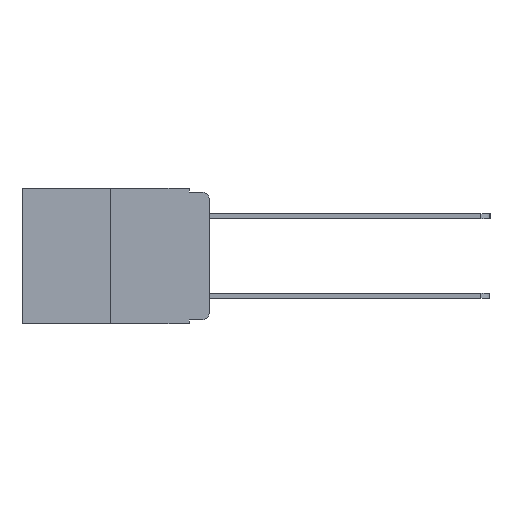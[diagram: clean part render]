
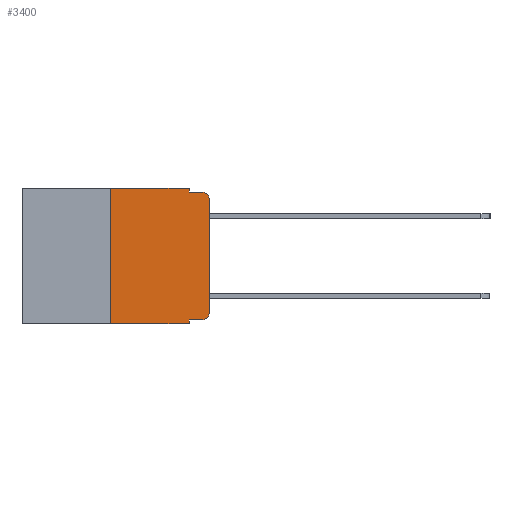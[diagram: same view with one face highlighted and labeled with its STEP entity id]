
A CAD part, left-side view. The second image highlights one B-rep face of the part: STEP entity #3400.
In plain terms, the highlighted planar face has unit normal (-1, 0, 0).
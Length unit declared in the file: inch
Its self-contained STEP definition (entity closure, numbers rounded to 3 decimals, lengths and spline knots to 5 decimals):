
#88 = ORIENTED_EDGE ( 'NONE', *, *, #11592, .F. ) ;
#136 = EDGE_LOOP ( 'NONE', ( #2099, #2999, #10190, #9305, #88, #3889, #4144, #408, #235, #6968 ) ) ;
#235 = ORIENTED_EDGE ( 'NONE', *, *, #1915, .T. ) ;
#408 = ORIENTED_EDGE ( 'NONE', *, *, #4943, .F. ) ;
#869 = VERTEX_POINT ( 'NONE', #4973 ) ;
#880 = VERTEX_POINT ( 'NONE', #2454 ) ;
#1146 = DIRECTION ( 'NONE',  ( 0., 0., 1. ) ) ;
#1280 = CARTESIAN_POINT ( 'NONE',  ( 0., 0.051, -0.01 ) ) ;
#1501 = CARTESIAN_POINT ( 'NONE',  ( 0., 0.02, -0.313 ) ) ;
#1856 = AXIS2_PLACEMENT_3D ( 'NONE', #10428, #14400, #14117 ) ;
#1915 = EDGE_CURVE ( 'NONE', #10577, #4329, #13606, .T. ) ;
#2099 = ORIENTED_EDGE ( 'NONE', *, *, #10039, .T. ) ;
#2454 = CARTESIAN_POINT ( 'NONE',  ( 0., 0.051, -0.01 ) ) ;
#2602 = VERTEX_POINT ( 'NONE', #11830 ) ;
#2999 = ORIENTED_EDGE ( 'NONE', *, *, #15874, .T. ) ;
#3044 = DIRECTION ( 'NONE',  ( 0., 0., -1. ) ) ;
#3115 = DIRECTION ( 'NONE',  ( 0., -1., 0. ) ) ;
#3323 = CARTESIAN_POINT ( 'NONE',  ( 0., 0.051, -0.333 ) ) ;
#3326 = VECTOR ( 'NONE', #14661, 39.37008 ) ;
#3400 = ADVANCED_FACE ( 'NONE', ( #4817 ), #15267, .F. ) ;
#3598 = LINE ( 'NONE', #12659, #15865 ) ;
#3889 = ORIENTED_EDGE ( 'NONE', *, *, #6284, .F. ) ;
#4144 = ORIENTED_EDGE ( 'NONE', *, *, #9678, .T. ) ;
#4246 = DIRECTION ( 'NONE',  ( 0., 0., -1. ) ) ;
#4329 = VERTEX_POINT ( 'NONE', #7805 ) ;
#4361 = CARTESIAN_POINT ( 'NONE',  ( 0., 0.02, -0.03 ) ) ;
#4480 = CIRCLE ( 'NONE', #6885, 0.02 ) ;
#4817 = FACE_OUTER_BOUND ( 'NONE', #136, .T. ) ;
#4943 = EDGE_CURVE ( 'NONE', #10577, #2602, #14174, .T. ) ;
#4973 = CARTESIAN_POINT ( 'NONE',  ( 0., 0.051, 0. ) ) ;
#5614 = DIRECTION ( 'NONE',  ( 0., 0., -1. ) ) ;
#5935 = CARTESIAN_POINT ( 'NONE',  ( 0., 0.051, -0.333 ) ) ;
#6029 = VECTOR ( 'NONE', #1146, 39.37008 ) ;
#6284 = EDGE_CURVE ( 'NONE', #9981, #15827, #15373, .T. ) ;
#6334 = EDGE_CURVE ( 'NONE', #880, #10778, #11234, .T. ) ;
#6389 = CARTESIAN_POINT ( 'NONE',  ( 0., 0.473, 0. ) ) ;
#6442 = DIRECTION ( 'NONE',  ( 0., -1., 0. ) ) ;
#6521 = VERTEX_POINT ( 'NONE', #14118 ) ;
#6801 = CARTESIAN_POINT ( 'NONE',  ( 0., 0.051, 0. ) ) ;
#6885 = AXIS2_PLACEMENT_3D ( 'NONE', #4361, #12760, #5614 ) ;
#6941 = CARTESIAN_POINT ( 'NONE',  ( 0., 0., -0.313 ) ) ;
#6968 = ORIENTED_EDGE ( 'NONE', *, *, #7679, .T. ) ;
#7152 = CARTESIAN_POINT ( 'NONE',  ( 0., 0., 0. ) ) ;
#7525 = VECTOR ( 'NONE', #13862, 39.37008 ) ;
#7598 = EDGE_CURVE ( 'NONE', #869, #880, #3598, .T. ) ;
#7645 = CARTESIAN_POINT ( 'NONE',  ( 0., 0.473, -0.343 ) ) ;
#7679 = EDGE_CURVE ( 'NONE', #4329, #13127, #9331, .T. ) ;
#7805 = CARTESIAN_POINT ( 'NONE',  ( 0., 0.02, -0.333 ) ) ;
#8067 = VECTOR ( 'NONE', #12635, 39.37008 ) ;
#8331 = DIRECTION ( 'NONE',  ( 0., 0., 1. ) ) ;
#9038 = VECTOR ( 'NONE', #6442, 39.37008 ) ;
#9305 = ORIENTED_EDGE ( 'NONE', *, *, #7598, .F. ) ;
#9331 = CIRCLE ( 'NONE', #14561, 0.02 ) ;
#9678 = EDGE_CURVE ( 'NONE', #9981, #2602, #15624, .T. ) ;
#9981 = VERTEX_POINT ( 'NONE', #11829 ) ;
#10039 = EDGE_CURVE ( 'NONE', #13127, #6521, #14721, .T. ) ;
#10190 = ORIENTED_EDGE ( 'NONE', *, *, #6334, .F. ) ;
#10428 = CARTESIAN_POINT ( 'NONE',  ( 0., 0.473, 0. ) ) ;
#10431 = DIRECTION ( 'NONE',  ( -1., 0., 0. ) ) ;
#10577 = VERTEX_POINT ( 'NONE', #5935 ) ;
#10778 = VERTEX_POINT ( 'NONE', #12359 ) ;
#11234 = LINE ( 'NONE', #1280, #8067 ) ;
#11592 = EDGE_CURVE ( 'NONE', #15827, #869, #12210, .T. ) ;
#11693 = VECTOR ( 'NONE', #8331, 39.37008 ) ;
#11829 = CARTESIAN_POINT ( 'NONE',  ( 0., 0.25, -0.343 ) ) ;
#11830 = CARTESIAN_POINT ( 'NONE',  ( 0., 0.051, -0.343 ) ) ;
#12210 = LINE ( 'NONE', #6389, #9038 ) ;
#12359 = CARTESIAN_POINT ( 'NONE',  ( 0., 0.02, -0.01 ) ) ;
#12635 = DIRECTION ( 'NONE',  ( 0., -1., 0. ) ) ;
#12659 = CARTESIAN_POINT ( 'NONE',  ( 0., 0.051, 0. ) ) ;
#12760 = DIRECTION ( 'NONE',  ( -1., 0., 0. ) ) ;
#13127 = VERTEX_POINT ( 'NONE', #6941 ) ;
#13250 = VECTOR ( 'NONE', #3115, 39.37008 ) ;
#13606 = LINE ( 'NONE', #3323, #13250 ) ;
#13862 = DIRECTION ( 'NONE',  ( 0., 0., -1. ) ) ;
#14117 = DIRECTION ( 'NONE',  ( 0., 0., -1. ) ) ;
#14118 = CARTESIAN_POINT ( 'NONE',  ( 0., 0., -0.03 ) ) ;
#14174 = LINE ( 'NONE', #6801, #7525 ) ;
#14400 = DIRECTION ( 'NONE',  ( 1., 0., 0. ) ) ;
#14561 = AXIS2_PLACEMENT_3D ( 'NONE', #1501, #10431, #3044 ) ;
#14661 = DIRECTION ( 'NONE',  ( 0., -1., 0. ) ) ;
#14721 = LINE ( 'NONE', #7152, #11693 ) ;
#14922 = CARTESIAN_POINT ( 'NONE',  ( 0., 0.25, 0. ) ) ;
#15267 = PLANE ( 'NONE',  #1856 ) ;
#15373 = LINE ( 'NONE', #15893, #6029 ) ;
#15624 = LINE ( 'NONE', #7645, #3326 ) ;
#15827 = VERTEX_POINT ( 'NONE', #14922 ) ;
#15865 = VECTOR ( 'NONE', #4246, 39.37008 ) ;
#15874 = EDGE_CURVE ( 'NONE', #6521, #10778, #4480, .T. ) ;
#15893 = CARTESIAN_POINT ( 'NONE',  ( 0., 0.25, 0. ) ) ;
